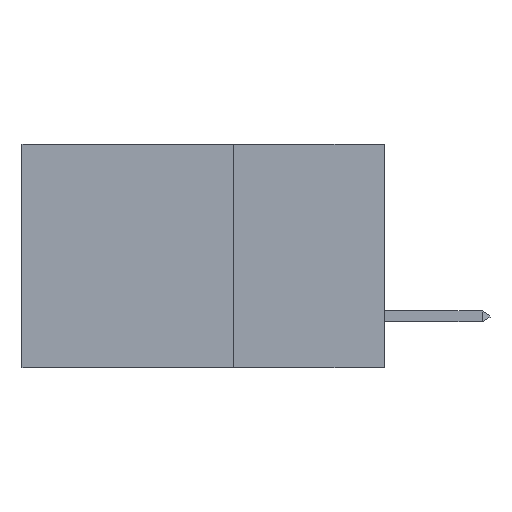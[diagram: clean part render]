
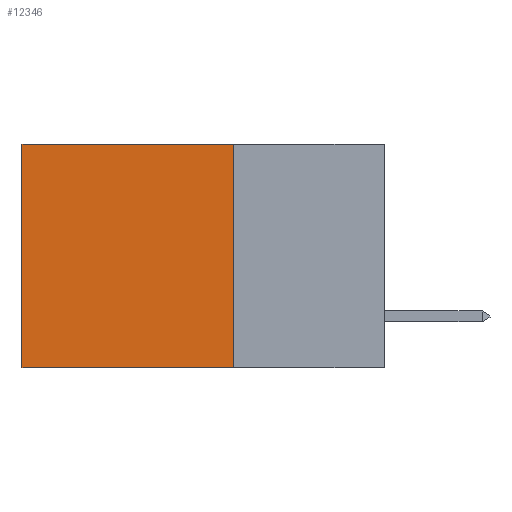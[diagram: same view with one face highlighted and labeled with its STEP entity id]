
A CAD part, left-side view. The second image highlights one B-rep face of the part: STEP entity #12346.
In plain terms, the highlighted planar face has unit normal (-1, 0, 0).
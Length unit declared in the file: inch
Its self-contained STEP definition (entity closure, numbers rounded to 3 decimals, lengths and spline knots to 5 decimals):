
#329 = DIRECTION ( 'NONE',  ( 0., 0., -1. ) ) ;
#534 = EDGE_CURVE ( 'NONE', #9102, #1572, #10829, .T. ) ;
#1148 = CARTESIAN_POINT ( 'NONE',  ( 0.2875, 0.25, 0. ) ) ;
#1243 = ORIENTED_EDGE ( 'NONE', *, *, #7820, .F. ) ;
#1572 = VERTEX_POINT ( 'NONE', #9392 ) ;
#1617 = VERTEX_POINT ( 'NONE', #10803 ) ;
#2245 = DIRECTION ( 'NONE',  ( 0., 1., 0. ) ) ;
#2247 = ORIENTED_EDGE ( 'NONE', *, *, #4560, .T. ) ;
#2462 = DIRECTION ( 'NONE',  ( 0., 0., -1. ) ) ;
#3149 = LINE ( 'NONE', #7987, #13300 ) ;
#3421 = LINE ( 'NONE', #1148, #8468 ) ;
#3570 = ORIENTED_EDGE ( 'NONE', *, *, #8113, .T. ) ;
#4560 = EDGE_CURVE ( 'NONE', #9102, #4891, #3421, .T. ) ;
#4891 = VERTEX_POINT ( 'NONE', #11364 ) ;
#5095 = CARTESIAN_POINT ( 'NONE',  ( 0.2875, 0.25, -0.37 ) ) ;
#5565 = AXIS2_PLACEMENT_3D ( 'NONE', #7853, #8896, #2462 ) ;
#6215 = LINE ( 'NONE', #5095, #11455 ) ;
#6791 = ORIENTED_EDGE ( 'NONE', *, *, #534, .F. ) ;
#6794 = PLANE ( 'NONE',  #5565 ) ;
#7563 = DIRECTION ( 'NONE',  ( 0., 0., -1. ) ) ;
#7820 = EDGE_CURVE ( 'NONE', #1572, #1617, #6215, .T. ) ;
#7853 = CARTESIAN_POINT ( 'NONE',  ( 0.2875, 0.25, 0. ) ) ;
#7987 = CARTESIAN_POINT ( 'NONE',  ( 0.2875, 0.6, 0. ) ) ;
#8113 = EDGE_CURVE ( 'NONE', #4891, #1617, #3149, .T. ) ;
#8468 = VECTOR ( 'NONE', #2245, 39.37008 ) ;
#8896 = DIRECTION ( 'NONE',  ( 1., 0., 0. ) ) ;
#9102 = VERTEX_POINT ( 'NONE', #10182 ) ;
#9136 = CARTESIAN_POINT ( 'NONE',  ( 0.2875, 0.25, 0. ) ) ;
#9392 = CARTESIAN_POINT ( 'NONE',  ( 0.2875, 0.25, -0.37 ) ) ;
#10182 = CARTESIAN_POINT ( 'NONE',  ( 0.2875, 0.25, 0. ) ) ;
#10803 = CARTESIAN_POINT ( 'NONE',  ( 0.2875, 0.6, -0.37 ) ) ;
#10829 = LINE ( 'NONE', #9136, #13775 ) ;
#11364 = CARTESIAN_POINT ( 'NONE',  ( 0.2875, 0.6, 0. ) ) ;
#11441 = DIRECTION ( 'NONE',  ( 0., 1., 0. ) ) ;
#11455 = VECTOR ( 'NONE', #11441, 39.37008 ) ;
#11826 = EDGE_LOOP ( 'NONE', ( #3570, #1243, #6791, #2247 ) ) ;
#12346 = ADVANCED_FACE ( 'NONE', ( #12421 ), #6794, .F. ) ;
#12421 = FACE_OUTER_BOUND ( 'NONE', #11826, .T. ) ;
#13300 = VECTOR ( 'NONE', #329, 39.37008 ) ;
#13775 = VECTOR ( 'NONE', #7563, 39.37008 ) ;
